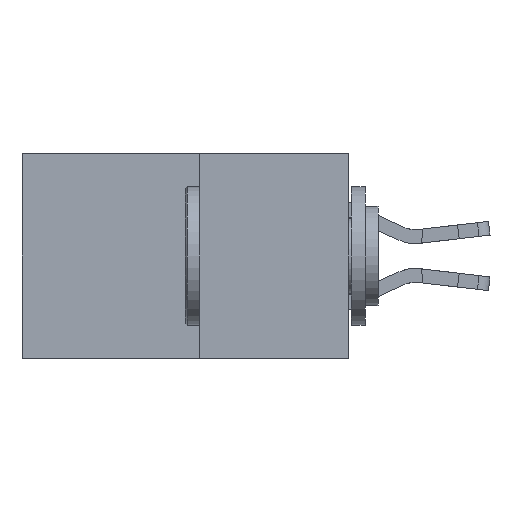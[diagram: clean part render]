
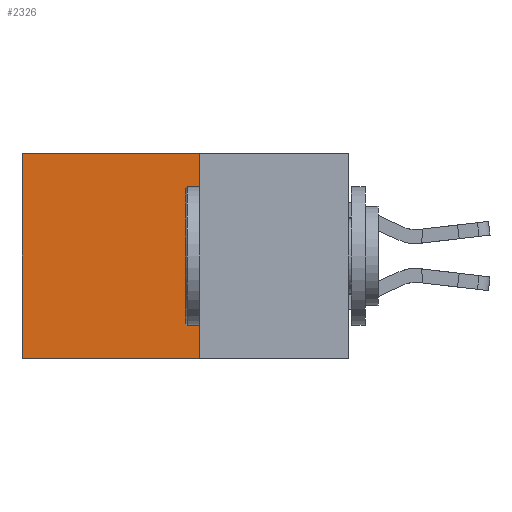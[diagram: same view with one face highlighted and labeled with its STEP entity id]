
A CAD part, left-side view. The second image highlights one B-rep face of the part: STEP entity #2326.
In plain terms, the highlighted planar face has unit normal (-1, 0, 0).
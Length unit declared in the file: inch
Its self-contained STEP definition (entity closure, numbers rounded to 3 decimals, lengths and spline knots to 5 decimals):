
#425 = LINE ( 'NONE', #11901, #12459 ) ;
#1151 = EDGE_LOOP ( 'NONE', ( #8526, #9586, #12104, #12131 ) ) ;
#1252 = CARTESIAN_POINT ( 'NONE',  ( 0.277, 0.27, -0.37 ) ) ;
#1402 = CARTESIAN_POINT ( 'NONE',  ( 0.277, 0.59, -0.37 ) ) ;
#1671 = LINE ( 'NONE', #10865, #7442 ) ;
#2326 = ADVANCED_FACE ( 'NONE', ( #4142 ), #10605, .F. ) ;
#2401 = VERTEX_POINT ( 'NONE', #1402 ) ;
#3195 = LINE ( 'NONE', #11313, #11513 ) ;
#4087 = EDGE_CURVE ( 'NONE', #5532, #9426, #3195, .T. ) ;
#4142 = FACE_OUTER_BOUND ( 'NONE', #1151, .T. ) ;
#4350 = LINE ( 'NONE', #6594, #9729 ) ;
#5529 = DIRECTION ( 'NONE',  ( 0., 1., 0. ) ) ;
#5532 = VERTEX_POINT ( 'NONE', #9353 ) ;
#6233 = EDGE_CURVE ( 'NONE', #5532, #6434, #425, .T. ) ;
#6360 = EDGE_CURVE ( 'NONE', #6434, #2401, #1671, .T. ) ;
#6434 = VERTEX_POINT ( 'NONE', #9998 ) ;
#6594 = CARTESIAN_POINT ( 'NONE',  ( 0.277, 0.59, -0.37 ) ) ;
#6710 = DIRECTION ( 'NONE',  ( 0., 0., -1. ) ) ;
#6882 = EDGE_CURVE ( 'NONE', #9426, #2401, #4350, .T. ) ;
#7442 = VECTOR ( 'NONE', #10832, 39.37008 ) ;
#8526 = ORIENTED_EDGE ( 'NONE', *, *, #6882, .T. ) ;
#9353 = CARTESIAN_POINT ( 'NONE',  ( 0.277, 0.27, 0. ) ) ;
#9426 = VERTEX_POINT ( 'NONE', #12728 ) ;
#9586 = ORIENTED_EDGE ( 'NONE', *, *, #6360, .F. ) ;
#9729 = VECTOR ( 'NONE', #6710, 39.37008 ) ;
#9998 = CARTESIAN_POINT ( 'NONE',  ( 0.277, 0.27, -0.37 ) ) ;
#10005 = DIRECTION ( 'NONE',  ( 1., 0., 0. ) ) ;
#10605 = PLANE ( 'NONE',  #14169 ) ;
#10764 = DIRECTION ( 'NONE',  ( 0., 0., -1. ) ) ;
#10832 = DIRECTION ( 'NONE',  ( 0., 1., 0. ) ) ;
#10865 = CARTESIAN_POINT ( 'NONE',  ( 0.277, 0.27, -0.37 ) ) ;
#11313 = CARTESIAN_POINT ( 'NONE',  ( 0.277, 0.27, 0. ) ) ;
#11513 = VECTOR ( 'NONE', #5529, 39.37008 ) ;
#11867 = DIRECTION ( 'NONE',  ( 0., 0., -1. ) ) ;
#11901 = CARTESIAN_POINT ( 'NONE',  ( 0.277, 0.27, -0.37 ) ) ;
#12104 = ORIENTED_EDGE ( 'NONE', *, *, #6233, .F. ) ;
#12131 = ORIENTED_EDGE ( 'NONE', *, *, #4087, .T. ) ;
#12459 = VECTOR ( 'NONE', #11867, 39.37008 ) ;
#12728 = CARTESIAN_POINT ( 'NONE',  ( 0.277, 0.59, 0. ) ) ;
#14169 = AXIS2_PLACEMENT_3D ( 'NONE', #1252, #10005, #10764 ) ;
